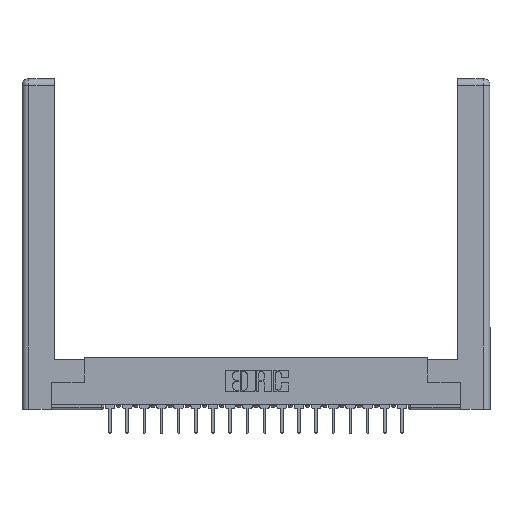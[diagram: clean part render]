
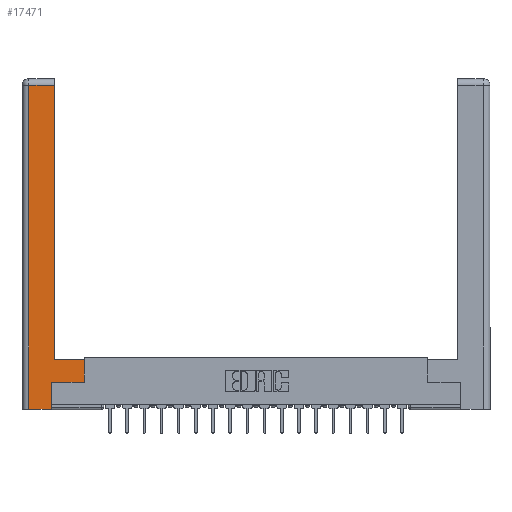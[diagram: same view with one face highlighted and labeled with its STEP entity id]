
A CAD part, top view. The second image highlights one B-rep face of the part: STEP entity #17471.
In plain terms, the highlighted planar face has unit normal (0, 0, 1).
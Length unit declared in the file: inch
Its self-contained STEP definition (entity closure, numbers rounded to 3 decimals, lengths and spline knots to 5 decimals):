
#202 = LINE ( 'NONE', #5629, #19719 ) ;
#1229 = LINE ( 'NONE', #1791, #2016 ) ;
#1488 = LINE ( 'NONE', #7466, #3331 ) ;
#1750 = VECTOR ( 'NONE', #8978, 39.37008 ) ;
#1791 = CARTESIAN_POINT ( 'NONE',  ( 0.265, 0., 0. ) ) ;
#2016 = VECTOR ( 'NONE', #11752, 39.37008 ) ;
#2331 = VECTOR ( 'NONE', #10891, 39.37008 ) ;
#2481 = VECTOR ( 'NONE', #9369, 39.37008 ) ;
#2935 = DIRECTION ( 'NONE',  ( -1., 0., 0. ) ) ;
#2991 = EDGE_CURVE ( 'NONE', #4723, #7409, #14808, .T. ) ;
#3290 = ORIENTED_EDGE ( 'NONE', *, *, #16491, .T. ) ;
#3331 = VECTOR ( 'NONE', #16051, 39.37008 ) ;
#4522 = CARTESIAN_POINT ( 'NONE',  ( 0.295, 2.94, 0. ) ) ;
#4723 = VERTEX_POINT ( 'NONE', #18990 ) ;
#5150 = ORIENTED_EDGE ( 'NONE', *, *, #5522, .T. ) ;
#5522 = EDGE_CURVE ( 'NONE', #8862, #20664, #6894, .T. ) ;
#5629 = CARTESIAN_POINT ( 'NONE',  ( 0.295, 3., 0. ) ) ;
#5806 = VECTOR ( 'NONE', #19918, 39.37008 ) ;
#6201 = PLANE ( 'NONE',  #16020 ) ;
#6457 = CARTESIAN_POINT ( 'NONE',  ( 0.265, 0., 0. ) ) ;
#6894 = LINE ( 'NONE', #19448, #2481 ) ;
#7409 = VERTEX_POINT ( 'NONE', #11426 ) ;
#7466 = CARTESIAN_POINT ( 'NONE',  ( 0.265, 0.245, 0. ) ) ;
#7593 = CARTESIAN_POINT ( 'NONE',  ( 0.0615, 0., 0. ) ) ;
#7679 = CARTESIAN_POINT ( 'NONE',  ( 0.565, 0.45, 0. ) ) ;
#7758 = EDGE_CURVE ( 'NONE', #16447, #11984, #1229, .T. ) ;
#7835 = DIRECTION ( 'NONE',  ( 0., 0., -1. ) ) ;
#7911 = EDGE_CURVE ( 'NONE', #18764, #8862, #202, .T. ) ;
#8064 = VECTOR ( 'NONE', #16042, 39.37008 ) ;
#8246 = CARTESIAN_POINT ( 'NONE',  ( 0.565, 0.245, 0. ) ) ;
#8728 = ORIENTED_EDGE ( 'NONE', *, *, #7758, .T. ) ;
#8862 = VERTEX_POINT ( 'NONE', #4522 ) ;
#8978 = DIRECTION ( 'NONE',  ( 0., -1., 0. ) ) ;
#9088 = CARTESIAN_POINT ( 'NONE',  ( 0.0615, 2.94, 0. ) ) ;
#9369 = DIRECTION ( 'NONE',  ( -1., 0., 0. ) ) ;
#10891 = DIRECTION ( 'NONE',  ( 0., 1., 0. ) ) ;
#11098 = CARTESIAN_POINT ( 'NONE',  ( 0.0615, 0., 0. ) ) ;
#11426 = CARTESIAN_POINT ( 'NONE',  ( 0.565, 0.45, 0. ) ) ;
#11752 = DIRECTION ( 'NONE',  ( 1., 0., 0. ) ) ;
#11829 = EDGE_CURVE ( 'NONE', #7409, #18764, #14837, .T. ) ;
#11984 = VERTEX_POINT ( 'NONE', #6457 ) ;
#13786 = ORIENTED_EDGE ( 'NONE', *, *, #2991, .T. ) ;
#14460 = CARTESIAN_POINT ( 'NONE',  ( 0., 0., 0. ) ) ;
#14808 = LINE ( 'NONE', #7679, #2331 ) ;
#14837 = LINE ( 'NONE', #19202, #8064 ) ;
#14984 = ORIENTED_EDGE ( 'NONE', *, *, #7911, .T. ) ;
#15293 = VERTEX_POINT ( 'NONE', #18421 ) ;
#16020 = AXIS2_PLACEMENT_3D ( 'NONE', #14460, #7835, #2935 ) ;
#16024 = CARTESIAN_POINT ( 'NONE',  ( 0.295, 0.45, 0. ) ) ;
#16042 = DIRECTION ( 'NONE',  ( -1., 0., 0. ) ) ;
#16044 = LINE ( 'NONE', #7593, #1750 ) ;
#16051 = DIRECTION ( 'NONE',  ( 0., 1., 0. ) ) ;
#16121 = ORIENTED_EDGE ( 'NONE', *, *, #21450, .T. ) ;
#16447 = VERTEX_POINT ( 'NONE', #11098 ) ;
#16491 = EDGE_CURVE ( 'NONE', #15293, #4723, #21187, .T. ) ;
#16613 = ORIENTED_EDGE ( 'NONE', *, *, #20066, .T. ) ;
#17201 = FACE_OUTER_BOUND ( 'NONE', #20970, .T. ) ;
#17471 = ADVANCED_FACE ( 'NONE', ( #17201 ), #6201, .F. ) ;
#18421 = CARTESIAN_POINT ( 'NONE',  ( 0.265, 0.245, 0. ) ) ;
#18764 = VERTEX_POINT ( 'NONE', #16024 ) ;
#18990 = CARTESIAN_POINT ( 'NONE',  ( 0.565, 0.245, 0. ) ) ;
#19202 = CARTESIAN_POINT ( 'NONE',  ( 0.295, 0.45, 0. ) ) ;
#19448 = CARTESIAN_POINT ( 'NONE',  ( 0.0615, 2.94, 0. ) ) ;
#19719 = VECTOR ( 'NONE', #20712, 39.37008 ) ;
#19918 = DIRECTION ( 'NONE',  ( 1., 0., 0. ) ) ;
#20026 = ORIENTED_EDGE ( 'NONE', *, *, #11829, .T. ) ;
#20066 = EDGE_CURVE ( 'NONE', #20664, #16447, #16044, .T. ) ;
#20664 = VERTEX_POINT ( 'NONE', #9088 ) ;
#20712 = DIRECTION ( 'NONE',  ( 0., 1., 0. ) ) ;
#20970 = EDGE_LOOP ( 'NONE', ( #14984, #5150, #16613, #8728, #16121, #3290, #13786, #20026 ) ) ;
#21187 = LINE ( 'NONE', #8246, #5806 ) ;
#21450 = EDGE_CURVE ( 'NONE', #11984, #15293, #1488, .T. ) ;
